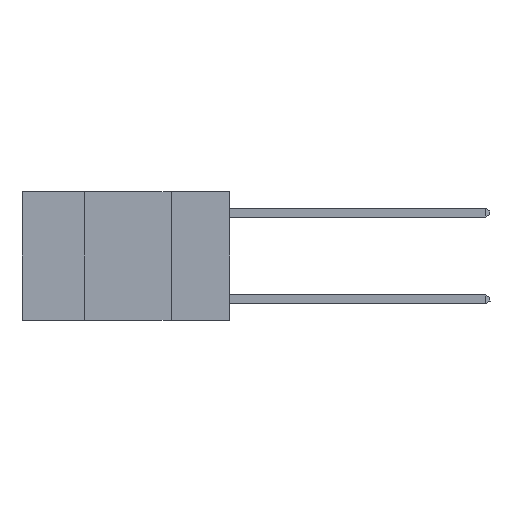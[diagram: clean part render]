
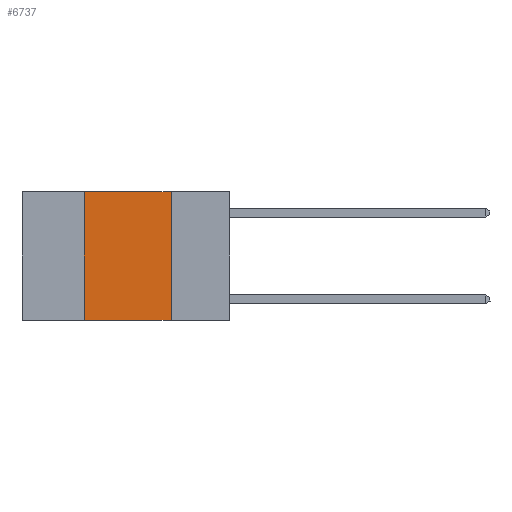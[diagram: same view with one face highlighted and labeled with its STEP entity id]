
A CAD part, left-side view. The second image highlights one B-rep face of the part: STEP entity #6737.
In plain terms, the highlighted planar face has unit normal (-1, 0, 0).
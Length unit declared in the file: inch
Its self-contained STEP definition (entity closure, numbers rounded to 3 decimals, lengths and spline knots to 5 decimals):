
#410 = LINE ( 'NONE', #1760, #12306 ) ;
#668 = CARTESIAN_POINT ( 'NONE',  ( 0., 0.6, 0. ) ) ;
#1407 = CARTESIAN_POINT ( 'NONE',  ( 0., 0.42, 0. ) ) ;
#1588 = CARTESIAN_POINT ( 'NONE',  ( 0., 0.17, 0. ) ) ;
#1760 = CARTESIAN_POINT ( 'NONE',  ( 0., 0.6, -0.37 ) ) ;
#1856 = DIRECTION ( 'NONE',  ( 0., 0., -1. ) ) ;
#1890 = ORIENTED_EDGE ( 'NONE', *, *, #4810, .F. ) ;
#2727 = CARTESIAN_POINT ( 'NONE',  ( 0., 0.6, 0. ) ) ;
#2729 = DIRECTION ( 'NONE',  ( 0., 0., -1. ) ) ;
#2957 = FACE_OUTER_BOUND ( 'NONE', #8555, .T. ) ;
#2966 = VERTEX_POINT ( 'NONE', #13106 ) ;
#4633 = VECTOR ( 'NONE', #12941, 39.37008 ) ;
#4751 = VERTEX_POINT ( 'NONE', #7684 ) ;
#4810 = EDGE_CURVE ( 'NONE', #9236, #2966, #14544, .T. ) ;
#5481 = ORIENTED_EDGE ( 'NONE', *, *, #10720, .F. ) ;
#6278 = DIRECTION ( 'NONE',  ( 0., 0., 1. ) ) ;
#6710 = AXIS2_PLACEMENT_3D ( 'NONE', #668, #9050, #1856 ) ;
#6737 = ADVANCED_FACE ( 'NONE', ( #2957 ), #14219, .F. ) ;
#6739 = VECTOR ( 'NONE', #2729, 39.37008 ) ;
#7684 = CARTESIAN_POINT ( 'NONE',  ( 0., 0.42, -0.37 ) ) ;
#7900 = LINE ( 'NONE', #2727, #4633 ) ;
#7992 = ORIENTED_EDGE ( 'NONE', *, *, #10172, .F. ) ;
#8411 = ORIENTED_EDGE ( 'NONE', *, *, #11875, .T. ) ;
#8555 = EDGE_LOOP ( 'NONE', ( #1890, #7992, #5481, #8411 ) ) ;
#9050 = DIRECTION ( 'NONE',  ( 1., 0., 0. ) ) ;
#9236 = VERTEX_POINT ( 'NONE', #11895 ) ;
#10172 = EDGE_CURVE ( 'NONE', #13347, #9236, #7900, .T. ) ;
#10469 = VECTOR ( 'NONE', #6278, 39.37008 ) ;
#10720 = EDGE_CURVE ( 'NONE', #4751, #13347, #13438, .T. ) ;
#11875 = EDGE_CURVE ( 'NONE', #4751, #2966, #410, .T. ) ;
#11895 = CARTESIAN_POINT ( 'NONE',  ( 0., 0.17, 0. ) ) ;
#12121 = DIRECTION ( 'NONE',  ( 0., -1., 0. ) ) ;
#12306 = VECTOR ( 'NONE', #12121, 39.37008 ) ;
#12748 = CARTESIAN_POINT ( 'NONE',  ( 0., 0.42, 0. ) ) ;
#12941 = DIRECTION ( 'NONE',  ( 0., -1., 0. ) ) ;
#13106 = CARTESIAN_POINT ( 'NONE',  ( 0., 0.17, -0.37 ) ) ;
#13347 = VERTEX_POINT ( 'NONE', #1407 ) ;
#13438 = LINE ( 'NONE', #12748, #10469 ) ;
#14219 = PLANE ( 'NONE',  #6710 ) ;
#14544 = LINE ( 'NONE', #1588, #6739 ) ;
